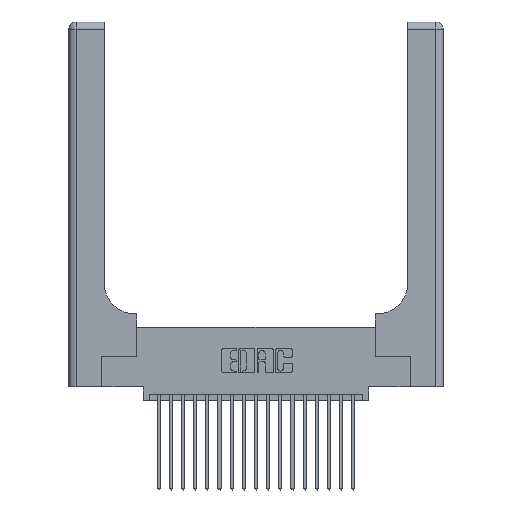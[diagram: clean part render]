
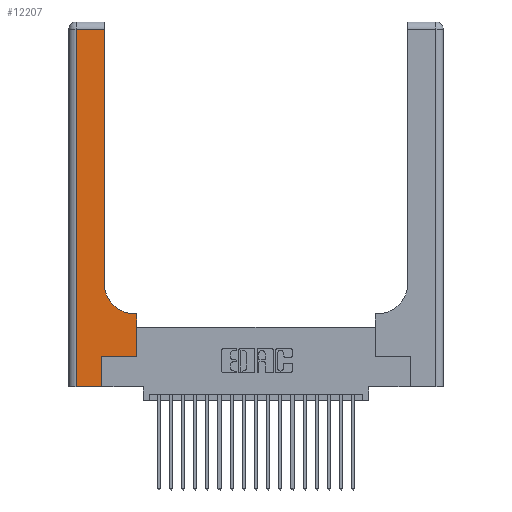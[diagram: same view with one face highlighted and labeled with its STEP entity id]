
A CAD part, top view. The second image highlights one B-rep face of the part: STEP entity #12207.
In plain terms, the highlighted planar face has unit normal (0, 0, 1).
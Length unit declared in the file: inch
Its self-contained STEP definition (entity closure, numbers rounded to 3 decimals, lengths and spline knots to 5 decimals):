
#183 = PLANE ( 'NONE',  #14016 ) ;
#297 = ORIENTED_EDGE ( 'NONE', *, *, #1185, .T. ) ;
#373 = CARTESIAN_POINT ( 'NONE',  ( 0.06, 0., 0.37 ) ) ;
#468 = LINE ( 'NONE', #11906, #9589 ) ;
#703 = VERTEX_POINT ( 'NONE', #3722 ) ;
#749 = LINE ( 'NONE', #7557, #18409 ) ;
#786 = CARTESIAN_POINT ( 'NONE',  ( 0.2915, 2.94, 0.37 ) ) ;
#1185 = EDGE_CURVE ( 'NONE', #1656, #13892, #749, .T. ) ;
#1656 = VERTEX_POINT ( 'NONE', #373 ) ;
#1710 = CARTESIAN_POINT ( 'NONE',  ( 0.269, 0., 0.37 ) ) ;
#2466 = CARTESIAN_POINT ( 'NONE',  ( 0.269, 0.25, 0.37 ) ) ;
#2675 = CARTESIAN_POINT ( 'NONE',  ( 0.2915, 0.85, 0.37 ) ) ;
#3354 = VECTOR ( 'NONE', #16281, 39.37008 ) ;
#3365 = DIRECTION ( 'NONE',  ( 0., 1., 0. ) ) ;
#3436 = DIRECTION ( 'NONE',  ( 0., 1., 0. ) ) ;
#3539 = DIRECTION ( 'NONE',  ( -1., 0., 0. ) ) ;
#3722 = CARTESIAN_POINT ( 'NONE',  ( 0.5415, 0.6, 0.37 ) ) ;
#3734 = EDGE_CURVE ( 'NONE', #19825, #1656, #11426, .T. ) ;
#4732 = CARTESIAN_POINT ( 'NONE',  ( 0.06, 3., 0.37 ) ) ;
#5142 = EDGE_LOOP ( 'NONE', ( #20829, #21345, #8911, #297, #15098, #18764, #14849, #11874, #16956 ) ) ;
#6369 = EDGE_CURVE ( 'NONE', #19477, #703, #16472, .T. ) ;
#6986 = CARTESIAN_POINT ( 'NONE',  ( 0., 2.94, 0.37 ) ) ;
#7100 = CARTESIAN_POINT ( 'NONE',  ( 0., 3., 0.37 ) ) ;
#7373 = DIRECTION ( 'NONE',  ( 1., 0., 0. ) ) ;
#7557 = CARTESIAN_POINT ( 'NONE',  ( 0., 0., 0.37 ) ) ;
#7575 = VERTEX_POINT ( 'NONE', #2675 ) ;
#8309 = VECTOR ( 'NONE', #3436, 39.37008 ) ;
#8826 = DIRECTION ( 'NONE',  ( -1., 0., 0. ) ) ;
#8911 = ORIENTED_EDGE ( 'NONE', *, *, #3734, .T. ) ;
#8936 = VECTOR ( 'NONE', #3539, 39.37008 ) ;
#8997 = VECTOR ( 'NONE', #17561, 39.37008 ) ;
#9376 = CARTESIAN_POINT ( 'NONE',  ( 0.269, 0., 0.37 ) ) ;
#9454 = LINE ( 'NONE', #6986, #8936 ) ;
#9588 = CARTESIAN_POINT ( 'NONE',  ( 0.5415, 0.85, 0.37 ) ) ;
#9589 = VECTOR ( 'NONE', #3365, 39.37008 ) ;
#10091 = CARTESIAN_POINT ( 'NONE',  ( 0.5585, 0.25, 0.37 ) ) ;
#10268 = EDGE_CURVE ( 'NONE', #16408, #19477, #19177, .T. ) ;
#10297 = EDGE_CURVE ( 'NONE', #7575, #16634, #468, .T. ) ;
#10308 = CIRCLE ( 'NONE', #12722, 0.25 ) ;
#10559 = CARTESIAN_POINT ( 'NONE',  ( 0.5585, 0.25, 0.37 ) ) ;
#11250 = FACE_OUTER_BOUND ( 'NONE', #5142, .T. ) ;
#11320 = DIRECTION ( 'NONE',  ( 1., 0., 0. ) ) ;
#11426 = LINE ( 'NONE', #4732, #15975 ) ;
#11874 = ORIENTED_EDGE ( 'NONE', *, *, #6369, .T. ) ;
#11906 = CARTESIAN_POINT ( 'NONE',  ( 0.2915, 3., 0.37 ) ) ;
#12109 = EDGE_CURVE ( 'NONE', #13892, #14452, #12857, .T. ) ;
#12207 = ADVANCED_FACE ( 'NONE', ( #11250 ), #183, .F. ) ;
#12722 = AXIS2_PLACEMENT_3D ( 'NONE', #9588, #21433, #11320 ) ;
#12857 = LINE ( 'NONE', #1710, #8309 ) ;
#13569 = DIRECTION ( 'NONE',  ( 0., 1., 0. ) ) ;
#13570 = LINE ( 'NONE', #15885, #8997 ) ;
#13892 = VERTEX_POINT ( 'NONE', #9376 ) ;
#14016 = AXIS2_PLACEMENT_3D ( 'NONE', #7100, #19005, #8826 ) ;
#14194 = VECTOR ( 'NONE', #13569, 39.37008 ) ;
#14452 = VERTEX_POINT ( 'NONE', #2466 ) ;
#14609 = CARTESIAN_POINT ( 'NONE',  ( 0.2915, 0.6, 0.37 ) ) ;
#14849 = ORIENTED_EDGE ( 'NONE', *, *, #10268, .T. ) ;
#15020 = DIRECTION ( 'NONE',  ( 0., -1., 0. ) ) ;
#15098 = ORIENTED_EDGE ( 'NONE', *, *, #12109, .T. ) ;
#15780 = CARTESIAN_POINT ( 'NONE',  ( 0.06, 2.94, 0.37 ) ) ;
#15885 = CARTESIAN_POINT ( 'NONE',  ( 0.269, 0.25, 0.37 ) ) ;
#15975 = VECTOR ( 'NONE', #15020, 39.37008 ) ;
#16050 = EDGE_CURVE ( 'NONE', #703, #7575, #10308, .T. ) ;
#16281 = DIRECTION ( 'NONE',  ( -1., 0., 0. ) ) ;
#16408 = VERTEX_POINT ( 'NONE', #10559 ) ;
#16472 = LINE ( 'NONE', #14609, #3354 ) ;
#16593 = CARTESIAN_POINT ( 'NONE',  ( 0.5585, 0.6, 0.37 ) ) ;
#16634 = VERTEX_POINT ( 'NONE', #786 ) ;
#16956 = ORIENTED_EDGE ( 'NONE', *, *, #16050, .T. ) ;
#17561 = DIRECTION ( 'NONE',  ( 1., 0., 0. ) ) ;
#18224 = EDGE_CURVE ( 'NONE', #14452, #16408, #13570, .T. ) ;
#18409 = VECTOR ( 'NONE', #7373, 39.37008 ) ;
#18764 = ORIENTED_EDGE ( 'NONE', *, *, #18224, .T. ) ;
#19005 = DIRECTION ( 'NONE',  ( 0., 0., -1. ) ) ;
#19177 = LINE ( 'NONE', #10091, #14194 ) ;
#19477 = VERTEX_POINT ( 'NONE', #16593 ) ;
#19825 = VERTEX_POINT ( 'NONE', #15780 ) ;
#20400 = EDGE_CURVE ( 'NONE', #16634, #19825, #9454, .T. ) ;
#20829 = ORIENTED_EDGE ( 'NONE', *, *, #10297, .T. ) ;
#21345 = ORIENTED_EDGE ( 'NONE', *, *, #20400, .T. ) ;
#21433 = DIRECTION ( 'NONE',  ( 0., 0., -1. ) ) ;
